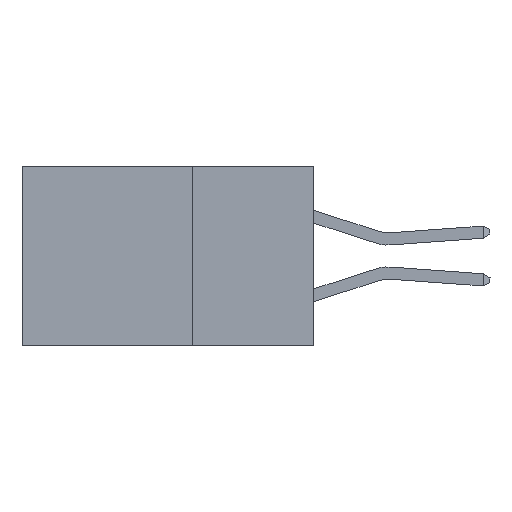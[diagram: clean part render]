
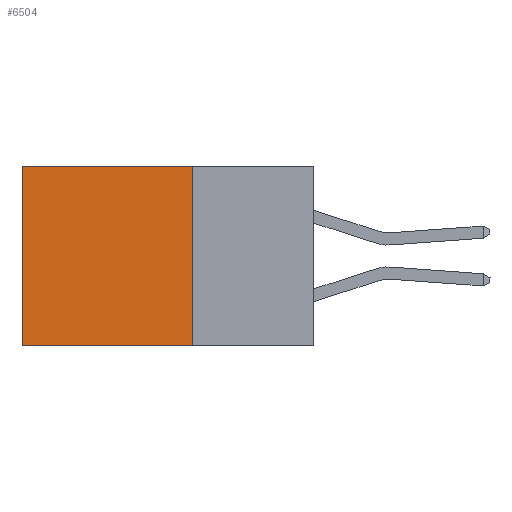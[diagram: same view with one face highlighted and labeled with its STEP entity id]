
A CAD part, left-side view. The second image highlights one B-rep face of the part: STEP entity #6504.
In plain terms, the highlighted planar face has unit normal (-1, 0, 0).
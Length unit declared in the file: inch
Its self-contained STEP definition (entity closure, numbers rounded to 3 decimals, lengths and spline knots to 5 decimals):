
#234 = CARTESIAN_POINT ( 'NONE',  ( 0.2875, 0.6, -0.37 ) ) ;
#1804 = CARTESIAN_POINT ( 'NONE',  ( 0.2875, 0.25, 0. ) ) ;
#3030 = VERTEX_POINT ( 'NONE', #234 ) ;
#3093 = EDGE_LOOP ( 'NONE', ( #28774, #12675, #7247, #23646 ) ) ;
#6168 = FACE_OUTER_BOUND ( 'NONE', #3093, .T. ) ;
#6504 = ADVANCED_FACE ( 'NONE', ( #6168 ), #10227, .F. ) ;
#7247 = ORIENTED_EDGE ( 'NONE', *, *, #11447, .F. ) ;
#7354 = VERTEX_POINT ( 'NONE', #28465 ) ;
#8252 = CARTESIAN_POINT ( 'NONE',  ( 0.2875, 0.25, -0.37 ) ) ;
#9789 = CARTESIAN_POINT ( 'NONE',  ( 0.2875, 0.25, 0. ) ) ;
#10227 = PLANE ( 'NONE',  #17455 ) ;
#11447 = EDGE_CURVE ( 'NONE', #7354, #23941, #26318, .T. ) ;
#12210 = CARTESIAN_POINT ( 'NONE',  ( 0.2875, 0.6, 0. ) ) ;
#12675 = ORIENTED_EDGE ( 'NONE', *, *, #25869, .F. ) ;
#12969 = EDGE_CURVE ( 'NONE', #7354, #15985, #27586, .T. ) ;
#13928 = DIRECTION ( 'NONE',  ( 0., 0., -1. ) ) ;
#14442 = DIRECTION ( 'NONE',  ( 0., 0., -1. ) ) ;
#15093 = DIRECTION ( 'NONE',  ( 0., 1., 0. ) ) ;
#15985 = VERTEX_POINT ( 'NONE', #12210 ) ;
#17455 = AXIS2_PLACEMENT_3D ( 'NONE', #21543, #23430, #23327 ) ;
#18244 = VECTOR ( 'NONE', #14442, 39.37008 ) ;
#19896 = DIRECTION ( 'NONE',  ( 0., 1., 0. ) ) ;
#20610 = CARTESIAN_POINT ( 'NONE',  ( 0.2875, 0.6, 0. ) ) ;
#21510 = VECTOR ( 'NONE', #15093, 39.37008 ) ;
#21543 = CARTESIAN_POINT ( 'NONE',  ( 0.2875, 0.25, 0. ) ) ;
#21654 = VECTOR ( 'NONE', #19896, 39.37008 ) ;
#22916 = LINE ( 'NONE', #8252, #21510 ) ;
#23327 = DIRECTION ( 'NONE',  ( 0., 0., -1. ) ) ;
#23430 = DIRECTION ( 'NONE',  ( 1., 0., 0. ) ) ;
#23646 = ORIENTED_EDGE ( 'NONE', *, *, #12969, .T. ) ;
#23941 = VERTEX_POINT ( 'NONE', #27265 ) ;
#25869 = EDGE_CURVE ( 'NONE', #23941, #3030, #22916, .T. ) ;
#26047 = VECTOR ( 'NONE', #13928, 39.37008 ) ;
#26318 = LINE ( 'NONE', #9789, #18244 ) ;
#27265 = CARTESIAN_POINT ( 'NONE',  ( 0.2875, 0.25, -0.37 ) ) ;
#27419 = LINE ( 'NONE', #20610, #26047 ) ;
#27465 = EDGE_CURVE ( 'NONE', #15985, #3030, #27419, .T. ) ;
#27586 = LINE ( 'NONE', #1804, #21654 ) ;
#28465 = CARTESIAN_POINT ( 'NONE',  ( 0.2875, 0.25, 0. ) ) ;
#28774 = ORIENTED_EDGE ( 'NONE', *, *, #27465, .T. ) ;
